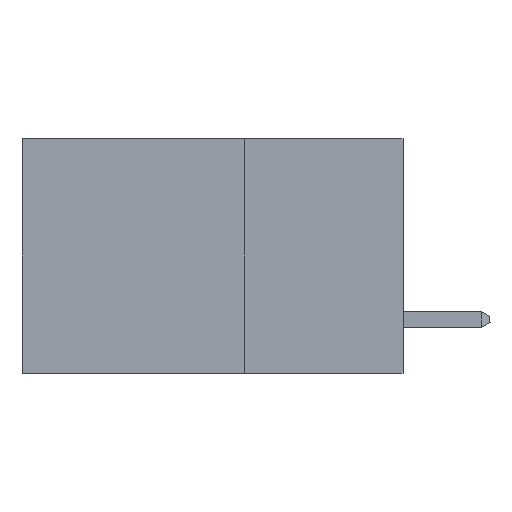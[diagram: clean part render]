
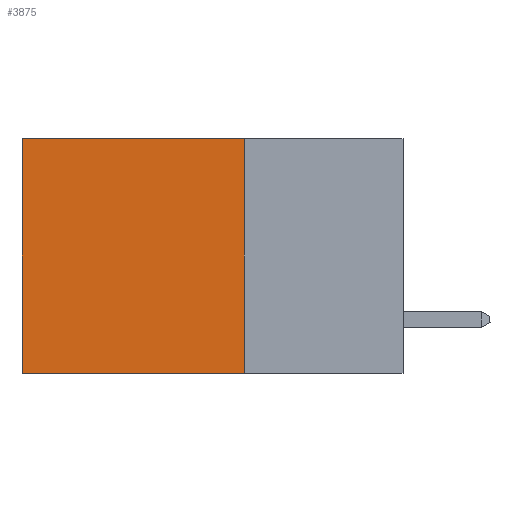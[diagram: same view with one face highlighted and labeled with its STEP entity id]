
A CAD part, left-side view. The second image highlights one B-rep face of the part: STEP entity #3875.
In plain terms, the highlighted planar face has unit normal (-1, 0, 0).
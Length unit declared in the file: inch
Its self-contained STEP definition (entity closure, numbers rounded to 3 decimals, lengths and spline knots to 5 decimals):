
#275 = LINE ( 'NONE', #817, #6285 ) ;
#817 = CARTESIAN_POINT ( 'NONE',  ( 0.2875, 0.25, -0.37 ) ) ;
#1113 = LINE ( 'NONE', #2716, #3352 ) ;
#1249 = VERTEX_POINT ( 'NONE', #6991 ) ;
#1320 = CARTESIAN_POINT ( 'NONE',  ( 0.2875, 0.25, -0.37 ) ) ;
#1341 = EDGE_CURVE ( 'NONE', #5570, #5730, #7030, .T. ) ;
#1898 = VERTEX_POINT ( 'NONE', #7045 ) ;
#1913 = CARTESIAN_POINT ( 'NONE',  ( 0.2875, 0.6, 0. ) ) ;
#2307 = CARTESIAN_POINT ( 'NONE',  ( 0.2875, 0.25, 0. ) ) ;
#2679 = CARTESIAN_POINT ( 'NONE',  ( 0.2875, 0.25, 0. ) ) ;
#2716 = CARTESIAN_POINT ( 'NONE',  ( 0.2875, 0.25, 0. ) ) ;
#3059 = FACE_OUTER_BOUND ( 'NONE', #4109, .T. ) ;
#3271 = DIRECTION ( 'NONE',  ( 0., 0., -1. ) ) ;
#3352 = VECTOR ( 'NONE', #5400, 39.37008 ) ;
#3619 = DIRECTION ( 'NONE',  ( 0., 0., -1. ) ) ;
#3875 = ADVANCED_FACE ( 'NONE', ( #3059 ), #7499, .F. ) ;
#3948 = LINE ( 'NONE', #1913, #5301 ) ;
#4017 = ORIENTED_EDGE ( 'NONE', *, *, #8412, .T. ) ;
#4109 = EDGE_LOOP ( 'NONE', ( #4017, #5377, #6798, #7941 ) ) ;
#5301 = VECTOR ( 'NONE', #3271, 39.37008 ) ;
#5377 = ORIENTED_EDGE ( 'NONE', *, *, #6476, .F. ) ;
#5400 = DIRECTION ( 'NONE',  ( 0., 1., 0. ) ) ;
#5570 = VERTEX_POINT ( 'NONE', #6572 ) ;
#5730 = VERTEX_POINT ( 'NONE', #1320 ) ;
#6285 = VECTOR ( 'NONE', #6824, 39.37008 ) ;
#6476 = EDGE_CURVE ( 'NONE', #5730, #1898, #275, .T. ) ;
#6572 = CARTESIAN_POINT ( 'NONE',  ( 0.2875, 0.25, 0. ) ) ;
#6798 = ORIENTED_EDGE ( 'NONE', *, *, #1341, .F. ) ;
#6824 = DIRECTION ( 'NONE',  ( 0., 1., 0. ) ) ;
#6891 = EDGE_CURVE ( 'NONE', #5570, #1249, #1113, .T. ) ;
#6991 = CARTESIAN_POINT ( 'NONE',  ( 0.2875, 0.6, 0. ) ) ;
#7030 = LINE ( 'NONE', #2307, #7558 ) ;
#7045 = CARTESIAN_POINT ( 'NONE',  ( 0.2875, 0.6, -0.37 ) ) ;
#7464 = DIRECTION ( 'NONE',  ( 0., 0., -1. ) ) ;
#7499 = PLANE ( 'NONE',  #7994 ) ;
#7558 = VECTOR ( 'NONE', #3619, 39.37008 ) ;
#7941 = ORIENTED_EDGE ( 'NONE', *, *, #6891, .T. ) ;
#7994 = AXIS2_PLACEMENT_3D ( 'NONE', #2679, #8075, #7464 ) ;
#8075 = DIRECTION ( 'NONE',  ( 1., 0., 0. ) ) ;
#8412 = EDGE_CURVE ( 'NONE', #1249, #1898, #3948, .T. ) ;
